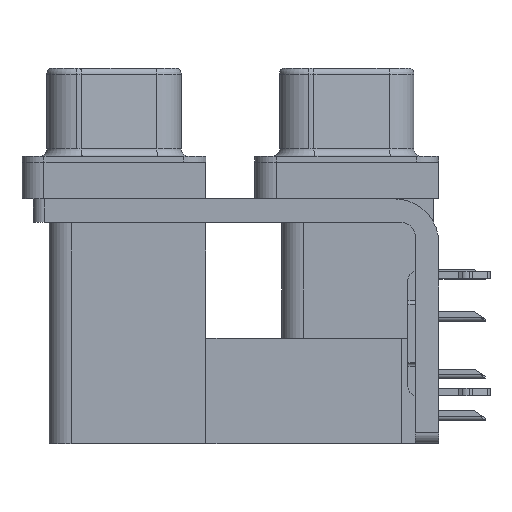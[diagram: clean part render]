
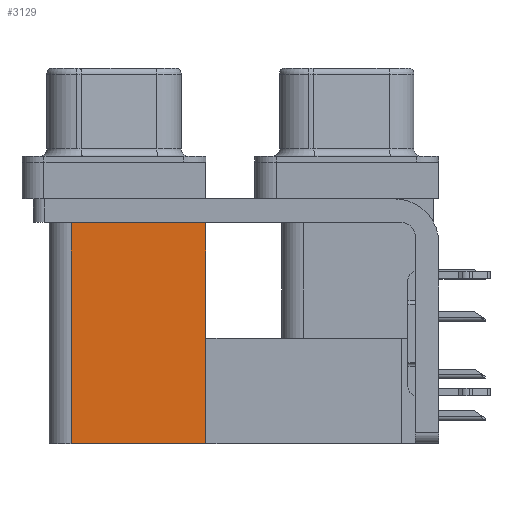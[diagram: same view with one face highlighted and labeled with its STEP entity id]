
A CAD part, left-side view. The second image highlights one B-rep face of the part: STEP entity #3129.
In plain terms, the highlighted planar face has unit normal (-1, 0, 0).
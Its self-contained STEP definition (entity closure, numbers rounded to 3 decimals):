
#458 = ORIENTED_EDGE ( 'NONE', *, *, #4560, .F. ) ;
#1764 = EDGE_CURVE ( 'NONE', #22568, #6387, #3221, .T. ) ;
#1945 = VECTOR ( 'NONE', #7726, 1000. ) ;
#2403 = CARTESIAN_POINT ( 'NONE',  ( 3.765, 9.6, -19.2 ) ) ;
#2849 = FACE_OUTER_BOUND ( 'NONE', #12900, .T. ) ;
#3129 = ADVANCED_FACE ( 'NONE', ( #2849 ), #12609, .F. ) ;
#3221 = LINE ( 'NONE', #12981, #28900 ) ;
#3858 = EDGE_CURVE ( 'NONE', #6387, #19453, #29460, .T. ) ;
#3873 = VECTOR ( 'NONE', #24135, 1000. ) ;
#4560 = EDGE_CURVE ( 'NONE', #27589, #19453, #8476, .T. ) ;
#6387 = VERTEX_POINT ( 'NONE', #18470 ) ;
#6397 = CARTESIAN_POINT ( 'NONE',  ( 3.765, 18.8, -19.2 ) ) ;
#7726 = DIRECTION ( 'NONE',  ( 0., 1., 0. ) ) ;
#8476 = LINE ( 'NONE', #6397, #17304 ) ;
#9107 = CARTESIAN_POINT ( 'NONE',  ( 3.765, 9.6, -19.2 ) ) ;
#10431 = CARTESIAN_POINT ( 'NONE',  ( 3.765, 9.6, -2.5 ) ) ;
#10876 = DIRECTION ( 'NONE',  ( 0., 0., 1. ) ) ;
#12566 = CARTESIAN_POINT ( 'NONE',  ( 3.765, 18.8, -19.2 ) ) ;
#12609 = PLANE ( 'NONE',  #25883 ) ;
#12671 = DIRECTION ( 'NONE',  ( 0., 0., 1. ) ) ;
#12900 = EDGE_LOOP ( 'NONE', ( #26361, #458, #27481, #30477 ) ) ;
#12981 = CARTESIAN_POINT ( 'NONE',  ( 3.765, 9.6, -19.2 ) ) ;
#15326 = DIRECTION ( 'NONE',  ( 1., 0., 0. ) ) ;
#17304 = VECTOR ( 'NONE', #10876, 1000. ) ;
#17725 = CARTESIAN_POINT ( 'NONE',  ( 3.765, 9.6, -19.2 ) ) ;
#18470 = CARTESIAN_POINT ( 'NONE',  ( 3.765, 9.6, -2.5 ) ) ;
#19453 = VERTEX_POINT ( 'NONE', #23050 ) ;
#22568 = VERTEX_POINT ( 'NONE', #9107 ) ;
#23050 = CARTESIAN_POINT ( 'NONE',  ( 3.765, 18.8, -2.5 ) ) ;
#24072 = EDGE_CURVE ( 'NONE', #22568, #27589, #26356, .T. ) ;
#24135 = DIRECTION ( 'NONE',  ( 0., 1., 0. ) ) ;
#25883 = AXIS2_PLACEMENT_3D ( 'NONE', #17725, #15326, #27454 ) ;
#26356 = LINE ( 'NONE', #2403, #3873 ) ;
#26361 = ORIENTED_EDGE ( 'NONE', *, *, #3858, .T. ) ;
#27454 = DIRECTION ( 'NONE',  ( 0., 0., -1. ) ) ;
#27481 = ORIENTED_EDGE ( 'NONE', *, *, #24072, .F. ) ;
#27589 = VERTEX_POINT ( 'NONE', #12566 ) ;
#28900 = VECTOR ( 'NONE', #12671, 1000. ) ;
#29460 = LINE ( 'NONE', #10431, #1945 ) ;
#30477 = ORIENTED_EDGE ( 'NONE', *, *, #1764, .T. ) ;
